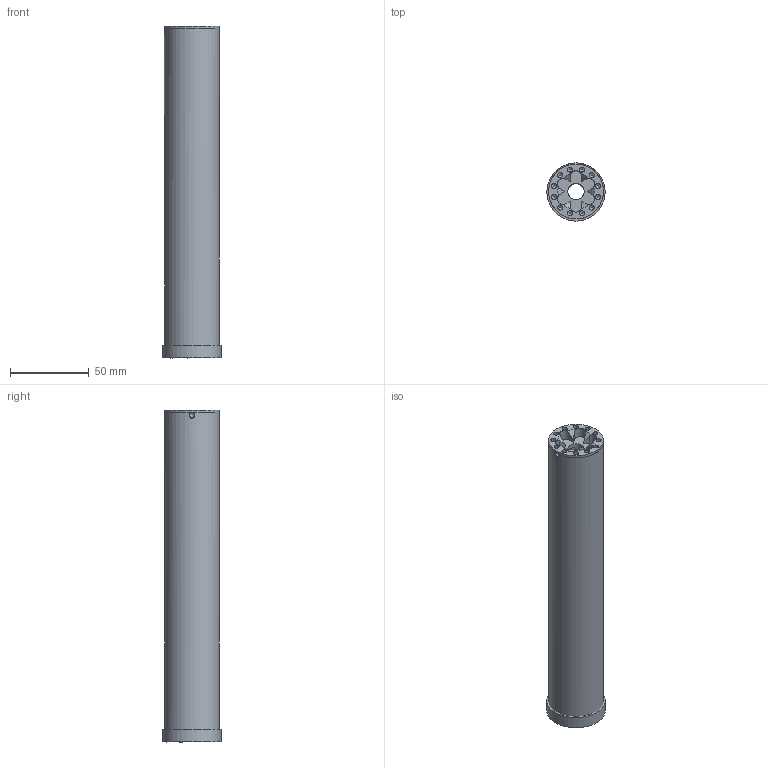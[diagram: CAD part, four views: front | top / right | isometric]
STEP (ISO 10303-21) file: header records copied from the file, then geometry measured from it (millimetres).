
FILE_DESCRIPTION (( 'STEP AP214' ), '1' );
FILE_NAME ('mystic clone assembly.step', '2016-02-01T19:15:30', ( 'WarFairy' ), ( '' ), 'SwSTEP 2.0', 'SolidWorks 2015', '' );
FILE_SCHEMA (( 'AUTOMOTIVE_DESIGN' ));
Length unit declared in the file: inch
Products named in the file (4): tube; core; mystic clone assembly; lockring
Assembly tree (3 placements, depth 2):
  mystic clone assembly
    core
    tube
    lockring
Bounding box: 37.08 x 37.08 x 211.28 mm (x, y, z)
Volume: 44244 mm3; surface area: 93540.5 mm2
Topology: 3 solids, 3 shells, 450 faces, 1377 edges, 910 vertices
Faces by surface type: cylinder 300, plane 125, cone 19, bspline 6
Full cylindrical faces by diameter (mm): 3.175 x13, 10.5 x11, 28.905 x12, 29.337 x1, 30.861 x3, 33.401 x18, 33.655 x1, 34.112 x1, 34.798 x1, 35.027 x1, 37.084 x1
Entity records: 22600 total; most frequent: CARTESIAN_POINT 12250, ORIENTED_EDGE 2366, DIRECTION 1718, EDGE_CURVE 1183, VERTEX_POINT 806, AXIS2_PLACEMENT_3D 616, EDGE_LOOP 519, LINE 486
